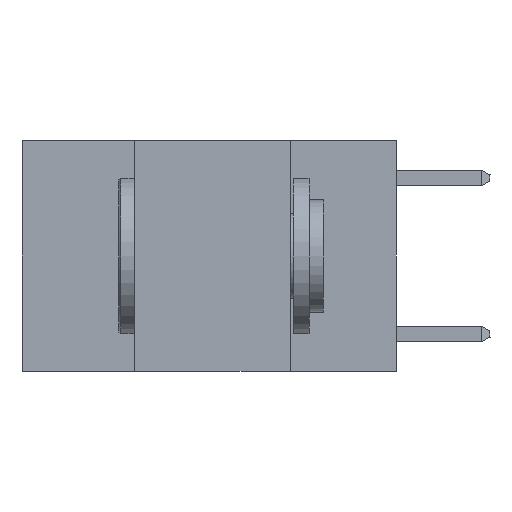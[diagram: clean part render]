
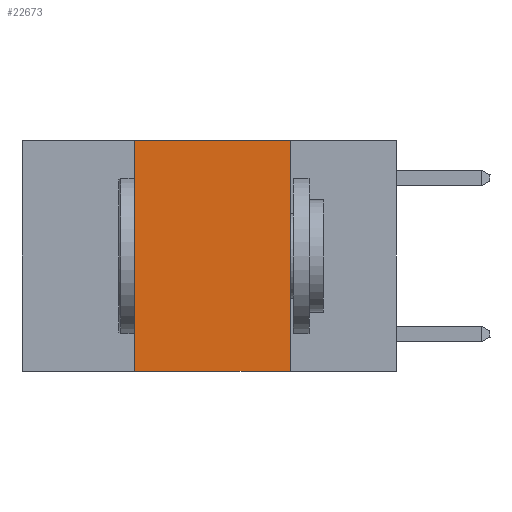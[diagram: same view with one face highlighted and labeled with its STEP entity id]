
A CAD part, left-side view. The second image highlights one B-rep face of the part: STEP entity #22673.
In plain terms, the highlighted planar face has unit normal (-1, 0, 0).
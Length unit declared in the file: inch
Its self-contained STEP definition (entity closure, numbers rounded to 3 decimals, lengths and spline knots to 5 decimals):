
#319 = LINE ( 'NONE', #2878, #2321 ) ;
#336 = VERTEX_POINT ( 'NONE', #2273 ) ;
#2075 = CARTESIAN_POINT ( 'NONE',  ( 0., 0.17, -0.37 ) ) ;
#2082 = LINE ( 'NONE', #9650, #21533 ) ;
#2273 = CARTESIAN_POINT ( 'NONE',  ( 0., 0.17, 0. ) ) ;
#2321 = VECTOR ( 'NONE', #2762, 39.37008 ) ;
#2565 = VERTEX_POINT ( 'NONE', #10966 ) ;
#2733 = DIRECTION ( 'NONE',  ( 1., 0., 0. ) ) ;
#2762 = DIRECTION ( 'NONE',  ( 0., -1., 0. ) ) ;
#2878 = CARTESIAN_POINT ( 'NONE',  ( 0., 0.6, -0.37 ) ) ;
#3355 = LINE ( 'NONE', #10912, #5726 ) ;
#3603 = DIRECTION ( 'NONE',  ( 0., 0., -1. ) ) ;
#4185 = EDGE_CURVE ( 'NONE', #2565, #13824, #319, .T. ) ;
#4237 = EDGE_CURVE ( 'NONE', #2565, #15241, #14059, .T. ) ;
#4678 = ORIENTED_EDGE ( 'NONE', *, *, #22810, .F. ) ;
#4750 = CARTESIAN_POINT ( 'NONE',  ( 0., 0.42, 0. ) ) ;
#5726 = VECTOR ( 'NONE', #24195, 39.37008 ) ;
#6927 = ORIENTED_EDGE ( 'NONE', *, *, #20475, .F. ) ;
#7437 = CARTESIAN_POINT ( 'NONE',  ( 0., 0.6, 0. ) ) ;
#8077 = AXIS2_PLACEMENT_3D ( 'NONE', #7437, #2733, #3603 ) ;
#9650 = CARTESIAN_POINT ( 'NONE',  ( 0., 0.17, 0. ) ) ;
#10912 = CARTESIAN_POINT ( 'NONE',  ( 0., 0.6, 0. ) ) ;
#10966 = CARTESIAN_POINT ( 'NONE',  ( 0., 0.42, -0.37 ) ) ;
#11410 = FACE_OUTER_BOUND ( 'NONE', #19041, .T. ) ;
#11691 = ORIENTED_EDGE ( 'NONE', *, *, #4237, .F. ) ;
#13598 = DIRECTION ( 'NONE',  ( 0., 0., 1. ) ) ;
#13824 = VERTEX_POINT ( 'NONE', #2075 ) ;
#14059 = LINE ( 'NONE', #4750, #21729 ) ;
#14142 = CARTESIAN_POINT ( 'NONE',  ( 0., 0.42, 0. ) ) ;
#15241 = VERTEX_POINT ( 'NONE', #14142 ) ;
#17245 = DIRECTION ( 'NONE',  ( 0., 0., -1. ) ) ;
#18875 = PLANE ( 'NONE',  #8077 ) ;
#19041 = EDGE_LOOP ( 'NONE', ( #6927, #4678, #11691, #23164 ) ) ;
#20475 = EDGE_CURVE ( 'NONE', #336, #13824, #2082, .T. ) ;
#21533 = VECTOR ( 'NONE', #17245, 39.37008 ) ;
#21729 = VECTOR ( 'NONE', #13598, 39.37008 ) ;
#22673 = ADVANCED_FACE ( 'NONE', ( #11410 ), #18875, .F. ) ;
#22810 = EDGE_CURVE ( 'NONE', #15241, #336, #3355, .T. ) ;
#23164 = ORIENTED_EDGE ( 'NONE', *, *, #4185, .T. ) ;
#24195 = DIRECTION ( 'NONE',  ( 0., -1., 0. ) ) ;
